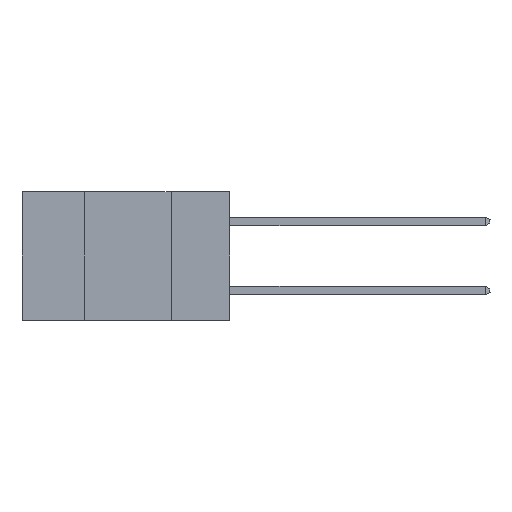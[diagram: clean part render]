
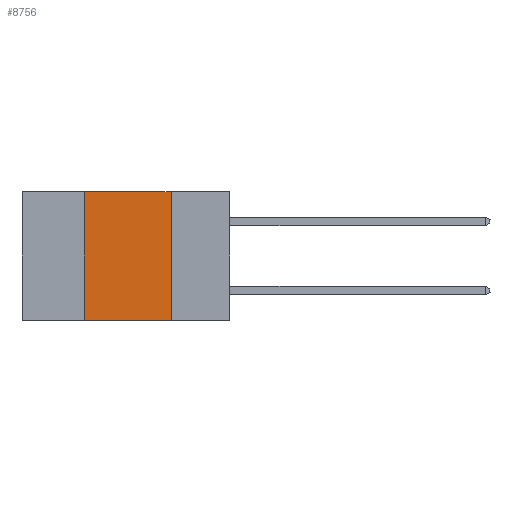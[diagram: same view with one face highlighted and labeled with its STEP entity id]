
A CAD part, left-side view. The second image highlights one B-rep face of the part: STEP entity #8756.
In plain terms, the highlighted planar face has unit normal (-1, 0, 0).
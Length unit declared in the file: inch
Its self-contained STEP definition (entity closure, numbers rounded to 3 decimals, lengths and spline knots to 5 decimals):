
#100 = DIRECTION ( 'NONE',  ( 0., -1., 0. ) ) ;
#481 = DIRECTION ( 'NONE',  ( 0., 0., -1. ) ) ;
#819 = VERTEX_POINT ( 'NONE', #7165 ) ;
#874 = VECTOR ( 'NONE', #3624, 39.37008 ) ;
#932 = VECTOR ( 'NONE', #481, 39.37008 ) ;
#1055 = CARTESIAN_POINT ( 'NONE',  ( 0., 0.42, 0. ) ) ;
#1483 = LINE ( 'NONE', #9011, #932 ) ;
#1912 = CARTESIAN_POINT ( 'NONE',  ( 0., 0.17, 0. ) ) ;
#1940 = EDGE_CURVE ( 'NONE', #3161, #7253, #1483, .T. ) ;
#2207 = ORIENTED_EDGE ( 'NONE', *, *, #7785, .F. ) ;
#2390 = FACE_OUTER_BOUND ( 'NONE', #10603, .T. ) ;
#2543 = LINE ( 'NONE', #6601, #3746 ) ;
#2675 = LINE ( 'NONE', #5309, #7730 ) ;
#3161 = VERTEX_POINT ( 'NONE', #1912 ) ;
#3199 = CARTESIAN_POINT ( 'NONE',  ( 0., 0.17, -0.37 ) ) ;
#3624 = DIRECTION ( 'NONE',  ( 0., 0., 1. ) ) ;
#3640 = DIRECTION ( 'NONE',  ( 0., 0., -1. ) ) ;
#3746 = VECTOR ( 'NONE', #7468, 39.37008 ) ;
#4415 = LINE ( 'NONE', #8433, #874 ) ;
#4665 = AXIS2_PLACEMENT_3D ( 'NONE', #7131, #7248, #3640 ) ;
#5309 = CARTESIAN_POINT ( 'NONE',  ( 0., 0.6, 0. ) ) ;
#5432 = ORIENTED_EDGE ( 'NONE', *, *, #1940, .F. ) ;
#6601 = CARTESIAN_POINT ( 'NONE',  ( 0., 0.6, -0.37 ) ) ;
#7131 = CARTESIAN_POINT ( 'NONE',  ( 0., 0.6, 0. ) ) ;
#7165 = CARTESIAN_POINT ( 'NONE',  ( 0., 0.42, -0.37 ) ) ;
#7248 = DIRECTION ( 'NONE',  ( 1., 0., 0. ) ) ;
#7253 = VERTEX_POINT ( 'NONE', #3199 ) ;
#7266 = ORIENTED_EDGE ( 'NONE', *, *, #9313, .F. ) ;
#7468 = DIRECTION ( 'NONE',  ( 0., -1., 0. ) ) ;
#7730 = VECTOR ( 'NONE', #100, 39.37008 ) ;
#7785 = EDGE_CURVE ( 'NONE', #8477, #3161, #2675, .T. ) ;
#8083 = PLANE ( 'NONE',  #4665 ) ;
#8433 = CARTESIAN_POINT ( 'NONE',  ( 0., 0.42, 0. ) ) ;
#8477 = VERTEX_POINT ( 'NONE', #1055 ) ;
#8756 = ADVANCED_FACE ( 'NONE', ( #2390 ), #8083, .F. ) ;
#8778 = ORIENTED_EDGE ( 'NONE', *, *, #10484, .T. ) ;
#9011 = CARTESIAN_POINT ( 'NONE',  ( 0., 0.17, 0. ) ) ;
#9313 = EDGE_CURVE ( 'NONE', #819, #8477, #4415, .T. ) ;
#10484 = EDGE_CURVE ( 'NONE', #819, #7253, #2543, .T. ) ;
#10603 = EDGE_LOOP ( 'NONE', ( #5432, #2207, #7266, #8778 ) ) ;
